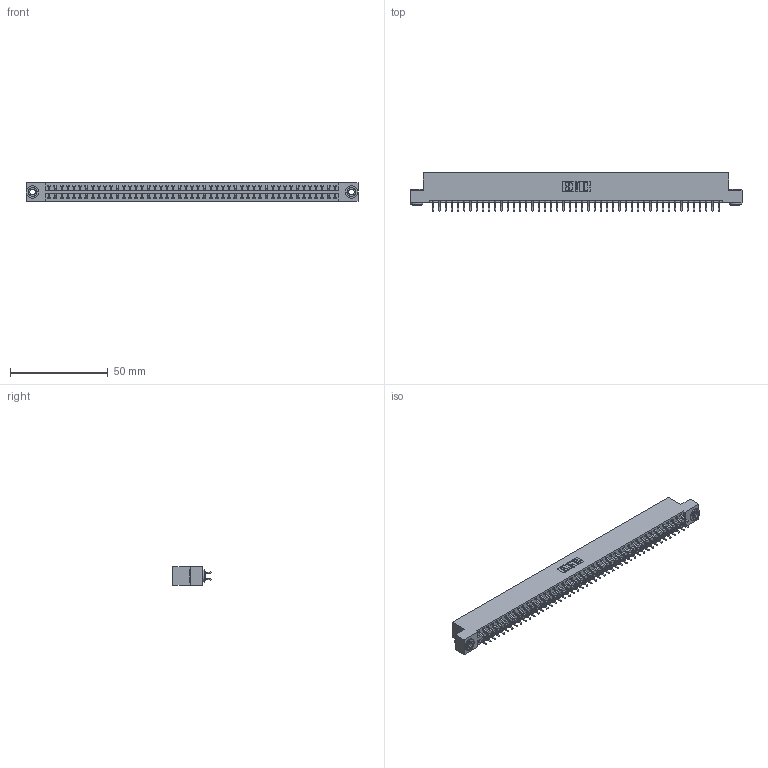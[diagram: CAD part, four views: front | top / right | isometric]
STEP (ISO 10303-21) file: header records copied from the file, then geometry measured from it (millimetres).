
FILE_DESCRIPTION (( 'STEP AP203' ), '1' );
FILE_NAME ('396-094-556-203.STEP', '2019-10-31T03:37:18', ( '' ), ( '' ), 'SwSTEP 2.0', 'SolidWorks 2016', '' );
FILE_SCHEMA (( 'CONFIG_CONTROL_DESIGN' ));
Length unit declared in the file: inch
Products named in the file (4): 345-250-002_345-250-002-102; 346 Part_Flush Mounting Lugs - 0.156 Dia-TH; 396-094-556-203; 345-292-001_556 Tail
Assembly tree (97 placements, depth 2):
  396-094-556-203
    346 Part_Flush Mounting Lugs - 0.156 Dia-TH
    345-292-001_556 Tail  x94
    345-250-002_345-250-002-102  x2
Bounding box: 169.8 x 19.57 x 9.4 mm (x, y, z)
Volume: 16612 mm3; surface area: 23039.8 mm2
Topology: 97 solids, 97 shells, 5612 faces, 16667 edges, 10982 vertices
Faces by surface type: plane 3752, cylinder 1852, cone 8
Entity records: 30870 total; most frequent: CARTESIAN_POINT 5071, ORIENTED_EDGE 4986, DIRECTION 4539, EDGE_CURVE 2493, VECTOR 2141, LINE 2141, VERTEX_POINT 1658, AXIS2_PLACEMENT_3D 1199
